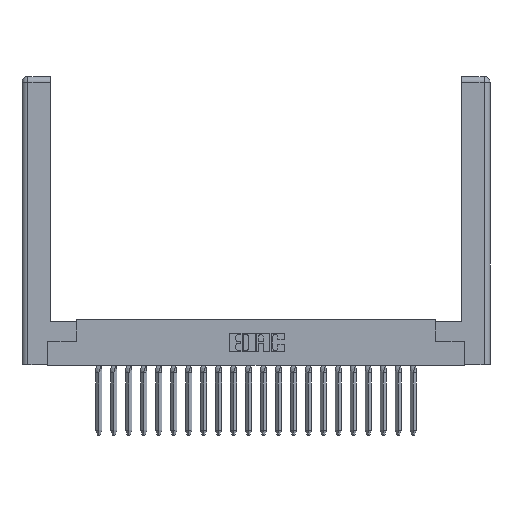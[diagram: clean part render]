
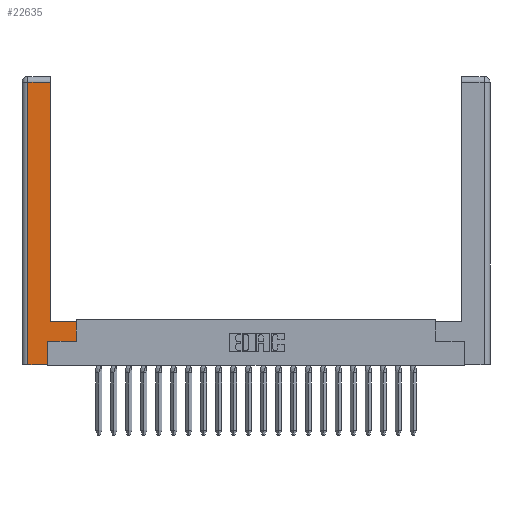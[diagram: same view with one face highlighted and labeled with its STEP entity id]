
A CAD part, top view. The second image highlights one B-rep face of the part: STEP entity #22635.
In plain terms, the highlighted planar face has unit normal (0, 0, 1).
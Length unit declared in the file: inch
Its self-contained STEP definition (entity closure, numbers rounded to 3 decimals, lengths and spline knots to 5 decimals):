
#24 = ORIENTED_EDGE ( 'NONE', *, *, #1913, .T. ) ;
#319 = LINE ( 'NONE', #23392, #30321 ) ;
#430 = CARTESIAN_POINT ( 'NONE',  ( 0.0615, 2.94, 0. ) ) ;
#1913 = EDGE_CURVE ( 'NONE', #20499, #45919, #319, .T. ) ;
#2327 = EDGE_CURVE ( 'NONE', #32872, #34298, #34258, .T. ) ;
#2353 = CARTESIAN_POINT ( 'NONE',  ( 0.565, 0.245, 0. ) ) ;
#2447 = PLANE ( 'NONE',  #34266 ) ;
#2593 = DIRECTION ( 'NONE',  ( 0., 0., -1. ) ) ;
#4637 = ORIENTED_EDGE ( 'NONE', *, *, #2327, .T. ) ;
#4753 = VERTEX_POINT ( 'NONE', #6063 ) ;
#5381 = VECTOR ( 'NONE', #16577, 39.37008 ) ;
#5604 = ORIENTED_EDGE ( 'NONE', *, *, #35766, .T. ) ;
#6063 = CARTESIAN_POINT ( 'NONE',  ( 0.295, 2.94, 0. ) ) ;
#6095 = CARTESIAN_POINT ( 'NONE',  ( 0., 0., 0. ) ) ;
#7635 = CARTESIAN_POINT ( 'NONE',  ( 0.0615, 2.94, 0. ) ) ;
#7651 = LINE ( 'NONE', #2353, #44981 ) ;
#8989 = DIRECTION ( 'NONE',  ( 1., 0., 0. ) ) ;
#9941 = ORIENTED_EDGE ( 'NONE', *, *, #45891, .T. ) ;
#10111 = EDGE_LOOP ( 'NONE', ( #9941, #36714, #24, #37418, #37391, #5604, #28728, #4637 ) ) ;
#11050 = CARTESIAN_POINT ( 'NONE',  ( 0.295, 0.45, 0. ) ) ;
#13644 = CARTESIAN_POINT ( 'NONE',  ( 0.565, 0.45, 0. ) ) ;
#14173 = VECTOR ( 'NONE', #26039, 39.37008 ) ;
#14221 = VECTOR ( 'NONE', #27421, 39.37008 ) ;
#16577 = DIRECTION ( 'NONE',  ( -1., 0., 0. ) ) ;
#17557 = LINE ( 'NONE', #22754, #39542 ) ;
#18024 = FACE_OUTER_BOUND ( 'NONE', #10111, .T. ) ;
#20499 = VERTEX_POINT ( 'NONE', #430 ) ;
#21136 = VECTOR ( 'NONE', #8989, 39.37008 ) ;
#22635 = ADVANCED_FACE ( 'NONE', ( #18024 ), #2447, .F. ) ;
#22754 = CARTESIAN_POINT ( 'NONE',  ( 0.295, 3., 0. ) ) ;
#22861 = CARTESIAN_POINT ( 'NONE',  ( 0.565, 0.45, 0. ) ) ;
#23392 = CARTESIAN_POINT ( 'NONE',  ( 0.0615, 0., 0. ) ) ;
#23909 = LINE ( 'NONE', #13644, #14221 ) ;
#25043 = CARTESIAN_POINT ( 'NONE',  ( 0.265, 0.245, 0. ) ) ;
#26039 = DIRECTION ( 'NONE',  ( -1., 0., 0. ) ) ;
#26754 = EDGE_CURVE ( 'NONE', #45919, #36921, #39718, .T. ) ;
#27267 = DIRECTION ( 'NONE',  ( 0., -1., 0. ) ) ;
#27421 = DIRECTION ( 'NONE',  ( 0., 1., 0. ) ) ;
#27952 = DIRECTION ( 'NONE',  ( -1., 0., 0. ) ) ;
#27990 = EDGE_CURVE ( 'NONE', #38465, #32872, #23909, .T. ) ;
#28728 = ORIENTED_EDGE ( 'NONE', *, *, #27990, .T. ) ;
#29765 = CARTESIAN_POINT ( 'NONE',  ( 0.0615, 0., 0. ) ) ;
#30277 = EDGE_CURVE ( 'NONE', #36921, #37583, #43356, .T. ) ;
#30321 = VECTOR ( 'NONE', #27267, 39.37008 ) ;
#31179 = CARTESIAN_POINT ( 'NONE',  ( 0.265, 0., 0. ) ) ;
#31446 = DIRECTION ( 'NONE',  ( 1., 0., 0. ) ) ;
#32872 = VERTEX_POINT ( 'NONE', #22861 ) ;
#33861 = DIRECTION ( 'NONE',  ( 0., 1., 0. ) ) ;
#34129 = CARTESIAN_POINT ( 'NONE',  ( 0.265, 0., 0. ) ) ;
#34258 = LINE ( 'NONE', #34551, #5381 ) ;
#34266 = AXIS2_PLACEMENT_3D ( 'NONE', #6095, #2593, #27952 ) ;
#34298 = VERTEX_POINT ( 'NONE', #11050 ) ;
#34551 = CARTESIAN_POINT ( 'NONE',  ( 0.295, 0.45, 0. ) ) ;
#35402 = DIRECTION ( 'NONE',  ( 0., 1., 0. ) ) ;
#35663 = LINE ( 'NONE', #7635, #14173 ) ;
#35766 = EDGE_CURVE ( 'NONE', #37583, #38465, #7651, .T. ) ;
#36706 = CARTESIAN_POINT ( 'NONE',  ( 0.565, 0.245, 0. ) ) ;
#36714 = ORIENTED_EDGE ( 'NONE', *, *, #45770, .T. ) ;
#36921 = VERTEX_POINT ( 'NONE', #31179 ) ;
#37391 = ORIENTED_EDGE ( 'NONE', *, *, #30277, .T. ) ;
#37418 = ORIENTED_EDGE ( 'NONE', *, *, #26754, .T. ) ;
#37583 = VERTEX_POINT ( 'NONE', #38543 ) ;
#38465 = VERTEX_POINT ( 'NONE', #36706 ) ;
#38543 = CARTESIAN_POINT ( 'NONE',  ( 0.265, 0.245, 0. ) ) ;
#39542 = VECTOR ( 'NONE', #33861, 39.37008 ) ;
#39718 = LINE ( 'NONE', #34129, #21136 ) ;
#42233 = VECTOR ( 'NONE', #35402, 39.37008 ) ;
#43356 = LINE ( 'NONE', #25043, #42233 ) ;
#44981 = VECTOR ( 'NONE', #31446, 39.37008 ) ;
#45770 = EDGE_CURVE ( 'NONE', #4753, #20499, #35663, .T. ) ;
#45891 = EDGE_CURVE ( 'NONE', #34298, #4753, #17557, .T. ) ;
#45919 = VERTEX_POINT ( 'NONE', #29765 ) ;
